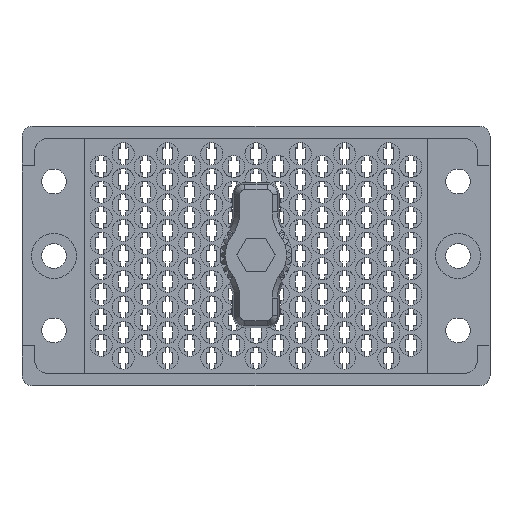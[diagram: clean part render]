
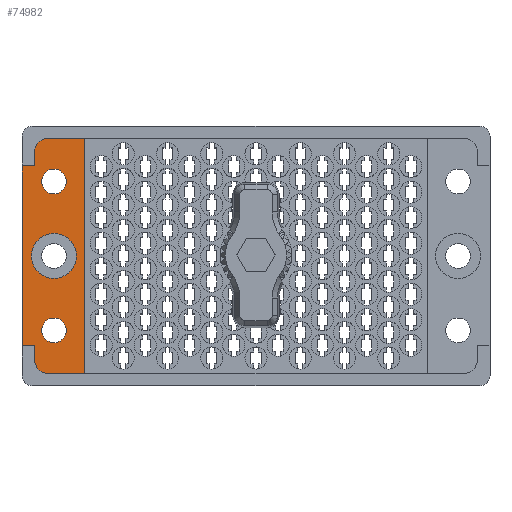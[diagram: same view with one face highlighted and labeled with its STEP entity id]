
A CAD part, top view. The second image highlights one B-rep face of the part: STEP entity #74982.
In plain terms, the highlighted planar face has unit normal (0, 0, 1).
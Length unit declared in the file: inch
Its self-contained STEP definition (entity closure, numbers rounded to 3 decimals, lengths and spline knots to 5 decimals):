
#294 = CIRCLE ( 'NONE', #77164, 0.0725 ) ;
#322 = VERTEX_POINT ( 'NONE', #91592 ) ;
#559 = FACE_BOUND ( 'NONE', #12271, .T. ) ;
#890 = AXIS2_PLACEMENT_3D ( 'NONE', #41688, #63986, #17995 ) ;
#962 = EDGE_CURVE ( 'NONE', #53573, #21527, #37365, .T. ) ;
#1308 = CARTESIAN_POINT ( 'NONE',  ( -1.3, 0., -0.117 ) ) ;
#2971 = EDGE_CURVE ( 'NONE', #58776, #30616, #294, .T. ) ;
#4080 = VERTEX_POINT ( 'NONE', #66323 ) ;
#7351 = EDGE_CURVE ( 'NONE', #4080, #46971, #34815, .T. ) ;
#7546 = CIRCLE ( 'NONE', #64890, 0.075 ) ;
#8497 = VECTOR ( 'NONE', #71004, 39.37008 ) ;
#8835 = ORIENTED_EDGE ( 'NONE', *, *, #81638, .T. ) ;
#9712 = CIRCLE ( 'NONE', #890, 0.1325 ) ;
#9863 = EDGE_CURVE ( 'NONE', #49158, #74307, #42026, .T. ) ;
#11959 = CARTESIAN_POINT ( 'NONE',  ( -1.375, 0.5285, -0.117 ) ) ;
#12271 = EDGE_LOOP ( 'NONE', ( #42490, #42835 ) ) ;
#12781 = CARTESIAN_POINT ( 'NONE',  ( -1.3, 0.5285, -0.117 ) ) ;
#13556 = DIRECTION ( 'NONE',  ( 0., 0., 1. ) ) ;
#13595 = DIRECTION ( 'NONE',  ( -1., 0., 0. ) ) ;
#15037 = VECTOR ( 'NONE', #55234, 39.37008 ) ;
#16003 = ORIENTED_EDGE ( 'NONE', *, *, #40796, .F. ) ;
#16837 = CARTESIAN_POINT ( 'NONE',  ( 0., -0.5285, -0.117 ) ) ;
#17458 = VERTEX_POINT ( 'NONE', #12781 ) ;
#17526 = CARTESIAN_POINT ( 'NONE',  ( -1.1875, 0.4375, -0.117 ) ) ;
#17995 = DIRECTION ( 'NONE',  ( 1., 0., 0. ) ) ;
#18854 = DIRECTION ( 'NONE',  ( 0., 0., 1. ) ) ;
#18882 = ORIENTED_EDGE ( 'NONE', *, *, #71940, .F. ) ;
#19949 = LINE ( 'NONE', #60014, #65963 ) ;
#21110 = ORIENTED_EDGE ( 'NONE', *, *, #2971, .F. ) ;
#21231 = FACE_BOUND ( 'NONE', #47833, .T. ) ;
#21527 = VERTEX_POINT ( 'NONE', #33725 ) ;
#22477 = VECTOR ( 'NONE', #51944, 39.37008 ) ;
#22982 = CIRCLE ( 'NONE', #27720, 0.075 ) ;
#23500 = DIRECTION ( 'NONE',  ( -1., 0., 0. ) ) ;
#23910 = VECTOR ( 'NONE', #79104, 39.37008 ) ;
#25126 = DIRECTION ( 'NONE',  ( 0., 0., 1. ) ) ;
#25780 = VERTEX_POINT ( 'NONE', #11959 ) ;
#27720 = AXIS2_PLACEMENT_3D ( 'NONE', #39128, #77461, #31019 ) ;
#28138 = CARTESIAN_POINT ( 'NONE',  ( -1.225, 0.615, -0.117 ) ) ;
#28701 = EDGE_LOOP ( 'NONE', ( #39766, #18882 ) ) ;
#30254 = ORIENTED_EDGE ( 'NONE', *, *, #94970, .F. ) ;
#30585 = ORIENTED_EDGE ( 'NONE', *, *, #88045, .F. ) ;
#30616 = VERTEX_POINT ( 'NONE', #57140 ) ;
#31019 = DIRECTION ( 'NONE',  ( 1., 0., 0. ) ) ;
#31501 = CIRCLE ( 'NONE', #100189, 0.0725 ) ;
#31579 = EDGE_CURVE ( 'NONE', #46971, #322, #19949, .T. ) ;
#33416 = EDGE_CURVE ( 'NONE', #17458, #25780, #91167, .T. ) ;
#33681 = PLANE ( 'NONE',  #63271 ) ;
#33725 = CARTESIAN_POINT ( 'NONE',  ( -1.115, 0.4375, -0.117 ) ) ;
#34406 = CARTESIAN_POINT ( 'NONE',  ( -1.1875, 0., -0.117 ) ) ;
#34815 = LINE ( 'NONE', #39466, #23910 ) ;
#37365 = CIRCLE ( 'NONE', #49102, 0.0725 ) ;
#38493 = VECTOR ( 'NONE', #94171, 39.37008 ) ;
#39128 = CARTESIAN_POINT ( 'NONE',  ( -1.225, -0.615, -0.117 ) ) ;
#39466 = CARTESIAN_POINT ( 'NONE',  ( -1.005, 0.7625, -0.117 ) ) ;
#39766 = ORIENTED_EDGE ( 'NONE', *, *, #962, .F. ) ;
#39956 = CARTESIAN_POINT ( 'NONE',  ( -1.3, 0., -0.117 ) ) ;
#40796 = EDGE_CURVE ( 'NONE', #30616, #58776, #71332, .T. ) ;
#41567 = DIRECTION ( 'NONE',  ( 0., 0., 1. ) ) ;
#41688 = CARTESIAN_POINT ( 'NONE',  ( -1.1875, 0., -0.117 ) ) ;
#42026 = CIRCLE ( 'NONE', #49656, 0.1325 ) ;
#42246 = CARTESIAN_POINT ( 'NONE',  ( -1.26, 0.4375, -0.117 ) ) ;
#42490 = ORIENTED_EDGE ( 'NONE', *, *, #43149, .F. ) ;
#42835 = ORIENTED_EDGE ( 'NONE', *, *, #9863, .F. ) ;
#43149 = EDGE_CURVE ( 'NONE', #74307, #49158, #9712, .T. ) ;
#44054 = EDGE_CURVE ( 'NONE', #78294, #73067, #22982, .T. ) ;
#44283 = AXIS2_PLACEMENT_3D ( 'NONE', #89889, #66732, #82749 ) ;
#45513 = LINE ( 'NONE', #66770, #22477 ) ;
#46689 = FACE_OUTER_BOUND ( 'NONE', #99345, .T. ) ;
#46971 = VERTEX_POINT ( 'NONE', #93115 ) ;
#47606 = VERTEX_POINT ( 'NONE', #71209 ) ;
#47833 = EDGE_LOOP ( 'NONE', ( #16003, #21110 ) ) ;
#48231 = ORIENTED_EDGE ( 'NONE', *, *, #7351, .T. ) ;
#49102 = AXIS2_PLACEMENT_3D ( 'NONE', #17526, #63530, #71345 ) ;
#49158 = VERTEX_POINT ( 'NONE', #80548 ) ;
#49656 = AXIS2_PLACEMENT_3D ( 'NONE', #34406, #18854, #57115 ) ;
#49715 = DIRECTION ( 'NONE',  ( 1., 0., 0. ) ) ;
#50602 = DIRECTION ( 'NONE',  ( 1., 0., 0. ) ) ;
#51118 = ORIENTED_EDGE ( 'NONE', *, *, #93629, .T. ) ;
#51178 = DIRECTION ( 'NONE',  ( 1., 0., 0. ) ) ;
#51944 = DIRECTION ( 'NONE',  ( -1., 0., 0. ) ) ;
#53341 = LINE ( 'NONE', #16837, #8497 ) ;
#53573 = VERTEX_POINT ( 'NONE', #42246 ) ;
#54330 = CARTESIAN_POINT ( 'NONE',  ( 0., 0.5285, -0.117 ) ) ;
#54433 = ORIENTED_EDGE ( 'NONE', *, *, #70284, .T. ) ;
#55234 = DIRECTION ( 'NONE',  ( 0., -1., 0. ) ) ;
#55921 = EDGE_CURVE ( 'NONE', #69587, #17458, #97956, .T. ) ;
#57115 = DIRECTION ( 'NONE',  ( 1., 0., 0. ) ) ;
#57140 = CARTESIAN_POINT ( 'NONE',  ( -1.26, -0.4375, -0.117 ) ) ;
#57820 = CARTESIAN_POINT ( 'NONE',  ( -1.1875, 0.4375, -0.117 ) ) ;
#58049 = ORIENTED_EDGE ( 'NONE', *, *, #31579, .T. ) ;
#58691 = LINE ( 'NONE', #1308, #15037 ) ;
#58753 = CARTESIAN_POINT ( 'NONE',  ( -1.3, 0.615, -0.117 ) ) ;
#58776 = VERTEX_POINT ( 'NONE', #84082 ) ;
#60014 = CARTESIAN_POINT ( 'NONE',  ( 0., 0.69, -0.117 ) ) ;
#63271 = AXIS2_PLACEMENT_3D ( 'NONE', #88596, #81138, #50602 ) ;
#63530 = DIRECTION ( 'NONE',  ( 0., 0., 1. ) ) ;
#63678 = CARTESIAN_POINT ( 'NONE',  ( -1.1875, -0.4375, -0.117 ) ) ;
#63986 = DIRECTION ( 'NONE',  ( 0., 0., 1. ) ) ;
#64890 = AXIS2_PLACEMENT_3D ( 'NONE', #28138, #13556, #51178 ) ;
#65963 = VECTOR ( 'NONE', #13595, 39.37008 ) ;
#66323 = CARTESIAN_POINT ( 'NONE',  ( -1.005, -0.69, -0.117 ) ) ;
#66732 = DIRECTION ( 'NONE',  ( 0., 0., 1. ) ) ;
#66770 = CARTESIAN_POINT ( 'NONE',  ( 0., -0.69, -0.117 ) ) ;
#67267 = FACE_BOUND ( 'NONE', #28701, .T. ) ;
#68904 = ORIENTED_EDGE ( 'NONE', *, *, #33416, .T. ) ;
#69587 = VERTEX_POINT ( 'NONE', #58753 ) ;
#69925 = DIRECTION ( 'NONE',  ( 0., -1., 0. ) ) ;
#70284 = EDGE_CURVE ( 'NONE', #322, #69587, #7546, .T. ) ;
#70819 = DIRECTION ( 'NONE',  ( 1., 0., 0. ) ) ;
#71004 = DIRECTION ( 'NONE',  ( -1., 0., 0. ) ) ;
#71209 = CARTESIAN_POINT ( 'NONE',  ( -1.3, -0.5285, -0.117 ) ) ;
#71332 = CIRCLE ( 'NONE', #44283, 0.0725 ) ;
#71345 = DIRECTION ( 'NONE',  ( 1., 0., 0. ) ) ;
#71543 = LINE ( 'NONE', #100202, #84936 ) ;
#71940 = EDGE_CURVE ( 'NONE', #21527, #53573, #31501, .T. ) ;
#72410 = ORIENTED_EDGE ( 'NONE', *, *, #44054, .T. ) ;
#73067 = VERTEX_POINT ( 'NONE', #100638 ) ;
#74307 = VERTEX_POINT ( 'NONE', #96514 ) ;
#74982 = ADVANCED_FACE ( 'NONE', ( #67267, #21231, #559, #46689 ), #33681, .T. ) ;
#77164 = AXIS2_PLACEMENT_3D ( 'NONE', #63678, #25126, #70819 ) ;
#77461 = DIRECTION ( 'NONE',  ( 0., 0., 1. ) ) ;
#78294 = VERTEX_POINT ( 'NONE', #89536 ) ;
#79104 = DIRECTION ( 'NONE',  ( 0., 1., 0. ) ) ;
#80548 = CARTESIAN_POINT ( 'NONE',  ( -1.32, 0., -0.117 ) ) ;
#80832 = CARTESIAN_POINT ( 'NONE',  ( -1.375, -0.5285, -0.117 ) ) ;
#80834 = VERTEX_POINT ( 'NONE', #80832 ) ;
#81138 = DIRECTION ( 'NONE',  ( 0., 0., 1. ) ) ;
#81638 = EDGE_CURVE ( 'NONE', #25780, #80834, #71543, .T. ) ;
#82700 = VECTOR ( 'NONE', #23500, 39.37008 ) ;
#82749 = DIRECTION ( 'NONE',  ( 1., 0., 0. ) ) ;
#84082 = CARTESIAN_POINT ( 'NONE',  ( -1.115, -0.4375, -0.117 ) ) ;
#84936 = VECTOR ( 'NONE', #69925, 39.37008 ) ;
#86550 = ORIENTED_EDGE ( 'NONE', *, *, #55921, .T. ) ;
#88045 = EDGE_CURVE ( 'NONE', #4080, #73067, #45513, .T. ) ;
#88596 = CARTESIAN_POINT ( 'NONE',  ( -1.375, -0.7625, -0.117 ) ) ;
#89536 = CARTESIAN_POINT ( 'NONE',  ( -1.3, -0.615, -0.117 ) ) ;
#89889 = CARTESIAN_POINT ( 'NONE',  ( -1.1875, -0.4375, -0.117 ) ) ;
#91167 = LINE ( 'NONE', #54330, #82700 ) ;
#91592 = CARTESIAN_POINT ( 'NONE',  ( -1.225, 0.69, -0.117 ) ) ;
#93115 = CARTESIAN_POINT ( 'NONE',  ( -1.005, 0.69, -0.117 ) ) ;
#93629 = EDGE_CURVE ( 'NONE', #47606, #78294, #58691, .T. ) ;
#94171 = DIRECTION ( 'NONE',  ( 0., -1., 0. ) ) ;
#94970 = EDGE_CURVE ( 'NONE', #47606, #80834, #53341, .T. ) ;
#96514 = CARTESIAN_POINT ( 'NONE',  ( -1.055, 0., -0.117 ) ) ;
#97956 = LINE ( 'NONE', #39956, #38493 ) ;
#99345 = EDGE_LOOP ( 'NONE', ( #58049, #54433, #86550, #68904, #8835, #30254, #51118, #72410, #30585, #48231 ) ) ;
#100189 = AXIS2_PLACEMENT_3D ( 'NONE', #57820, #41567, #49715 ) ;
#100202 = CARTESIAN_POINT ( 'NONE',  ( -1.375, 0.7625, -0.117 ) ) ;
#100638 = CARTESIAN_POINT ( 'NONE',  ( -1.225, -0.69, -0.117 ) ) ;
